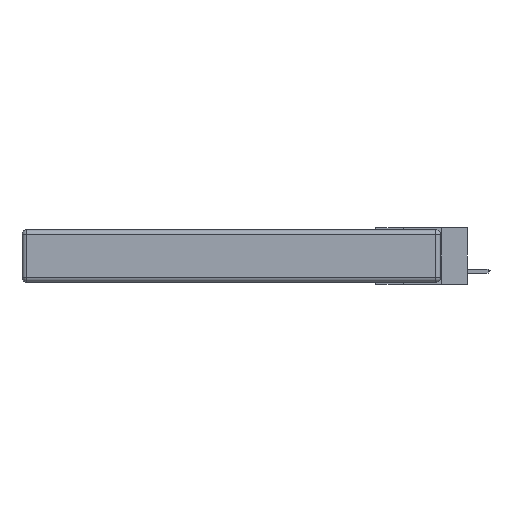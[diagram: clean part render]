
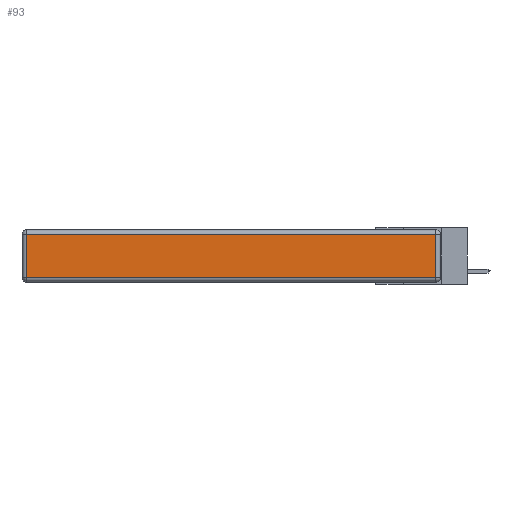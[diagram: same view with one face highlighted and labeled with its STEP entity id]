
A CAD part, left-side view. The second image highlights one B-rep face of the part: STEP entity #93.
In plain terms, the highlighted planar face has unit normal (-1, 0, 0).
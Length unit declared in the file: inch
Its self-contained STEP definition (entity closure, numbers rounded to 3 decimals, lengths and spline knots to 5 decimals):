
#93 = ADVANCED_FACE ( 'NONE', ( #4206 ), #10957, .T. ) ;
#267 = ORIENTED_EDGE ( 'NONE', *, *, #6034, .T. ) ;
#843 = EDGE_CURVE ( 'NONE', #1310, #11079, #1176, .T. ) ;
#882 = DIRECTION ( 'NONE',  ( 0., 1., 0. ) ) ;
#1176 = LINE ( 'NONE', #2709, #7559 ) ;
#1310 = VERTEX_POINT ( 'NONE', #1508 ) ;
#1508 = CARTESIAN_POINT ( 'NONE',  ( 0., 2.72, -0.313 ) ) ;
#1950 = CARTESIAN_POINT ( 'NONE',  ( 0., 0.03, -0.03 ) ) ;
#2168 = VECTOR ( 'NONE', #5757, 39.37008 ) ;
#2470 = LINE ( 'NONE', #3900, #2168 ) ;
#2660 = DIRECTION ( 'NONE',  ( 0., -1., 0. ) ) ;
#2709 = CARTESIAN_POINT ( 'NONE',  ( 0., 0., -0.313 ) ) ;
#3735 = LINE ( 'NONE', #3938, #10024 ) ;
#3900 = CARTESIAN_POINT ( 'NONE',  ( 0., 2.72, -0.343 ) ) ;
#3938 = CARTESIAN_POINT ( 'NONE',  ( 0., 2.75, -0.03 ) ) ;
#4206 = FACE_OUTER_BOUND ( 'NONE', #9919, .T. ) ;
#5757 = DIRECTION ( 'NONE',  ( 0., 0., -1. ) ) ;
#6034 = EDGE_CURVE ( 'NONE', #12162, #8426, #3735, .T. ) ;
#6039 = CARTESIAN_POINT ( 'NONE',  ( 0., 0., -0.343 ) ) ;
#6601 = EDGE_CURVE ( 'NONE', #11079, #12162, #11097, .T. ) ;
#7162 = ORIENTED_EDGE ( 'NONE', *, *, #7881, .T. ) ;
#7559 = VECTOR ( 'NONE', #2660, 39.37008 ) ;
#7881 = EDGE_CURVE ( 'NONE', #8426, #1310, #2470, .T. ) ;
#8010 = DIRECTION ( 'NONE',  ( -1., 0., 0. ) ) ;
#8151 = VECTOR ( 'NONE', #12453, 39.37008 ) ;
#8426 = VERTEX_POINT ( 'NONE', #12462 ) ;
#8461 = CARTESIAN_POINT ( 'NONE',  ( 0., 0.03, -0.313 ) ) ;
#8468 = ORIENTED_EDGE ( 'NONE', *, *, #6601, .T. ) ;
#9424 = CARTESIAN_POINT ( 'NONE',  ( 0., 0.03, -0.343 ) ) ;
#9919 = EDGE_LOOP ( 'NONE', ( #12270, #8468, #267, #7162 ) ) ;
#10003 = DIRECTION ( 'NONE',  ( 0., 0., 1. ) ) ;
#10024 = VECTOR ( 'NONE', #882, 39.37008 ) ;
#10957 = PLANE ( 'NONE',  #12174 ) ;
#11079 = VERTEX_POINT ( 'NONE', #8461 ) ;
#11097 = LINE ( 'NONE', #9424, #8151 ) ;
#12162 = VERTEX_POINT ( 'NONE', #1950 ) ;
#12174 = AXIS2_PLACEMENT_3D ( 'NONE', #6039, #8010, #10003 ) ;
#12270 = ORIENTED_EDGE ( 'NONE', *, *, #843, .T. ) ;
#12453 = DIRECTION ( 'NONE',  ( 0., 0., 1. ) ) ;
#12462 = CARTESIAN_POINT ( 'NONE',  ( 0., 2.72, -0.03 ) ) ;
